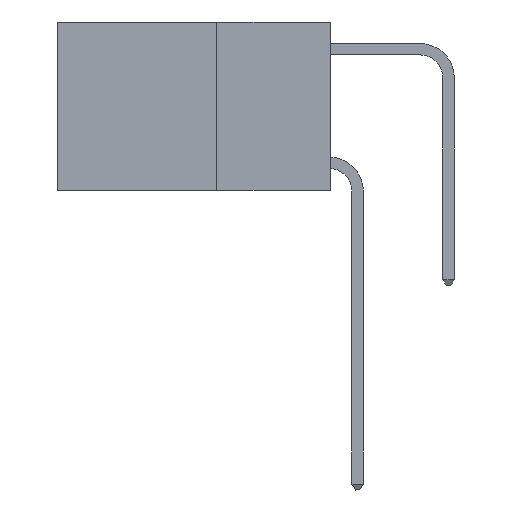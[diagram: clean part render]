
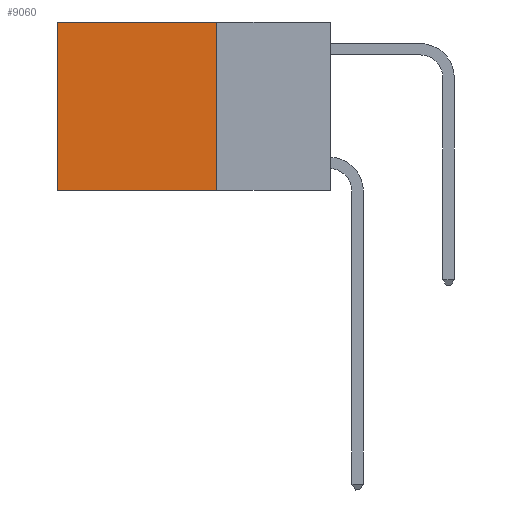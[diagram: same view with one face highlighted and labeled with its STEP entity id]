
A CAD part, left-side view. The second image highlights one B-rep face of the part: STEP entity #9060.
In plain terms, the highlighted planar face has unit normal (-1, 0, 0).
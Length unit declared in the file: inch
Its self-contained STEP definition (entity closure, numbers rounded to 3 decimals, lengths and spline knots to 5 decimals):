
#96 = EDGE_CURVE ( 'NONE', #12578, #27335, #1990, .T. ) ;
#735 = CARTESIAN_POINT ( 'NONE',  ( 0.2625, 0.25, -0.37 ) ) ;
#1990 = LINE ( 'NONE', #18633, #20804 ) ;
#3915 = DIRECTION ( 'NONE',  ( 0., 0., -1. ) ) ;
#6967 = LINE ( 'NONE', #14140, #23720 ) ;
#7262 = VERTEX_POINT ( 'NONE', #735 ) ;
#7563 = EDGE_CURVE ( 'NONE', #10225, #12578, #28186, .T. ) ;
#8523 = DIRECTION ( 'NONE',  ( 0., 0., -1. ) ) ;
#8550 = EDGE_CURVE ( 'NONE', #10225, #7262, #26794, .T. ) ;
#8726 = VECTOR ( 'NONE', #8523, 39.37008 ) ;
#9060 = ADVANCED_FACE ( 'NONE', ( #13431 ), #21296, .F. ) ;
#10225 = VERTEX_POINT ( 'NONE', #12012 ) ;
#10963 = CARTESIAN_POINT ( 'NONE',  ( 0.2625, 0.6, 0. ) ) ;
#11498 = VECTOR ( 'NONE', #28140, 39.37008 ) ;
#11904 = ORIENTED_EDGE ( 'NONE', *, *, #96, .T. ) ;
#12012 = CARTESIAN_POINT ( 'NONE',  ( 0.2625, 0.25, 0. ) ) ;
#12402 = ORIENTED_EDGE ( 'NONE', *, *, #7563, .T. ) ;
#12559 = CARTESIAN_POINT ( 'NONE',  ( 0.2625, 0.25, 0. ) ) ;
#12578 = VERTEX_POINT ( 'NONE', #10963 ) ;
#13091 = ORIENTED_EDGE ( 'NONE', *, *, #17861, .F. ) ;
#13431 = FACE_OUTER_BOUND ( 'NONE', #13462, .T. ) ;
#13462 = EDGE_LOOP ( 'NONE', ( #11904, #13091, #20941, #12402 ) ) ;
#14140 = CARTESIAN_POINT ( 'NONE',  ( 0.2625, 0.25, -0.37 ) ) ;
#15084 = CARTESIAN_POINT ( 'NONE',  ( 0.2625, 0.25, 0. ) ) ;
#16340 = DIRECTION ( 'NONE',  ( 0., 1., 0. ) ) ;
#16984 = DIRECTION ( 'NONE',  ( 1., 0., 0. ) ) ;
#17861 = EDGE_CURVE ( 'NONE', #7262, #27335, #6967, .T. ) ;
#18531 = DIRECTION ( 'NONE',  ( 0., 0., -1. ) ) ;
#18633 = CARTESIAN_POINT ( 'NONE',  ( 0.2625, 0.6, 0. ) ) ;
#18932 = AXIS2_PLACEMENT_3D ( 'NONE', #12559, #16984, #3915 ) ;
#19186 = CARTESIAN_POINT ( 'NONE',  ( 0.2625, 0.6, -0.37 ) ) ;
#19418 = CARTESIAN_POINT ( 'NONE',  ( 0.2625, 0.25, 0. ) ) ;
#20804 = VECTOR ( 'NONE', #18531, 39.37008 ) ;
#20941 = ORIENTED_EDGE ( 'NONE', *, *, #8550, .F. ) ;
#21296 = PLANE ( 'NONE',  #18932 ) ;
#23720 = VECTOR ( 'NONE', #16340, 39.37008 ) ;
#26794 = LINE ( 'NONE', #19418, #8726 ) ;
#27335 = VERTEX_POINT ( 'NONE', #19186 ) ;
#28140 = DIRECTION ( 'NONE',  ( 0., 1., 0. ) ) ;
#28186 = LINE ( 'NONE', #15084, #11498 ) ;
